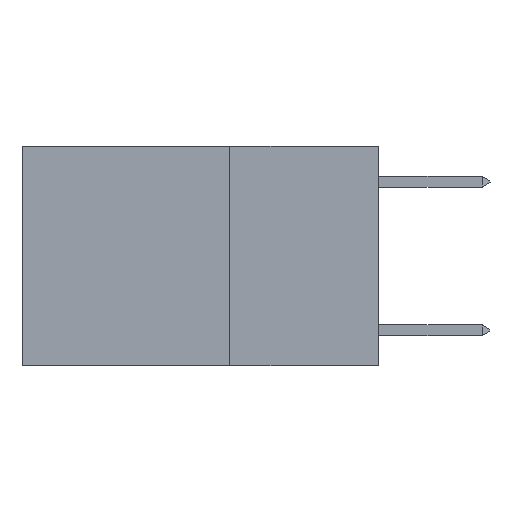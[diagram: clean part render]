
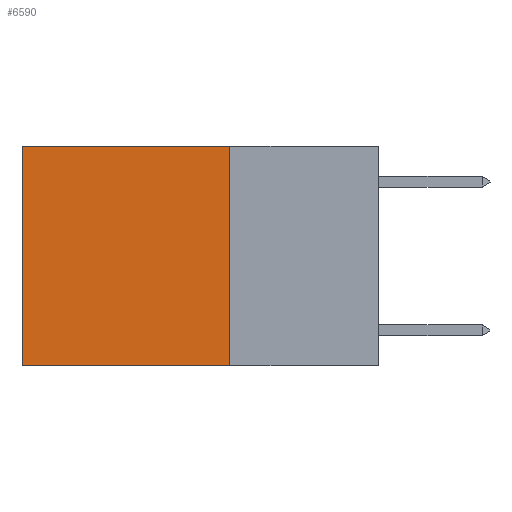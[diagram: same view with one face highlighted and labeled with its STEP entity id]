
A CAD part, left-side view. The second image highlights one B-rep face of the part: STEP entity #6590.
In plain terms, the highlighted planar face has unit normal (-1, 0, 0).
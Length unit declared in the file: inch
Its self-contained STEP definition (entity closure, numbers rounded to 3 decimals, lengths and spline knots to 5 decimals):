
#102 = LINE ( 'NONE', #12764, #19102 ) ;
#215 = EDGE_CURVE ( 'NONE', #3475, #6264, #17519, .T. ) ;
#253 = DIRECTION ( 'NONE',  ( 0., 0., -1. ) ) ;
#854 = LINE ( 'NONE', #14206, #12635 ) ;
#1300 = EDGE_LOOP ( 'NONE', ( #3783, #3819, #3892, #3922 ) ) ;
#2796 = CARTESIAN_POINT ( 'NONE',  ( 0.2625, 0.25, -0.37 ) ) ;
#3475 = VERTEX_POINT ( 'NONE', #7904 ) ;
#3783 = ORIENTED_EDGE ( 'NONE', *, *, #9590, .T. ) ;
#3819 = ORIENTED_EDGE ( 'NONE', *, *, #7355, .F. ) ;
#3892 = ORIENTED_EDGE ( 'NONE', *, *, #215, .F. ) ;
#3922 = ORIENTED_EDGE ( 'NONE', *, *, #8526, .T. ) ;
#4860 = FACE_OUTER_BOUND ( 'NONE', #1300, .T. ) ;
#5751 = DIRECTION ( 'NONE',  ( 0., 0., -1. ) ) ;
#6264 = VERTEX_POINT ( 'NONE', #2796 ) ;
#6590 = ADVANCED_FACE ( 'NONE', ( #4860 ), #16104, .F. ) ;
#7022 = CARTESIAN_POINT ( 'NONE',  ( 0.2625, 0.25, 0. ) ) ;
#7355 = EDGE_CURVE ( 'NONE', #6264, #15429, #854, .T. ) ;
#7838 = CARTESIAN_POINT ( 'NONE',  ( 0.2625, 0.25, 0. ) ) ;
#7904 = CARTESIAN_POINT ( 'NONE',  ( 0.2625, 0.25, 0. ) ) ;
#8027 = DIRECTION ( 'NONE',  ( 0., 1., 0. ) ) ;
#8526 = EDGE_CURVE ( 'NONE', #3475, #14657, #102, .T. ) ;
#8603 = DIRECTION ( 'NONE',  ( 1., 0., 0. ) ) ;
#9590 = EDGE_CURVE ( 'NONE', #14657, #15429, #19271, .T. ) ;
#11129 = VECTOR ( 'NONE', #5751, 39.37008 ) ;
#12266 = CARTESIAN_POINT ( 'NONE',  ( 0.2625, 0.6, -0.37 ) ) ;
#12592 = CARTESIAN_POINT ( 'NONE',  ( 0.2625, 0.6, 0. ) ) ;
#12635 = VECTOR ( 'NONE', #8027, 39.37008 ) ;
#12764 = CARTESIAN_POINT ( 'NONE',  ( 0.2625, 0.25, 0. ) ) ;
#13262 = VECTOR ( 'NONE', #253, 39.37008 ) ;
#14206 = CARTESIAN_POINT ( 'NONE',  ( 0.2625, 0.25, -0.37 ) ) ;
#14657 = VERTEX_POINT ( 'NONE', #12592 ) ;
#14951 = CARTESIAN_POINT ( 'NONE',  ( 0.2625, 0.6, 0. ) ) ;
#15429 = VERTEX_POINT ( 'NONE', #12266 ) ;
#15673 = DIRECTION ( 'NONE',  ( 0., 1., 0. ) ) ;
#16104 = PLANE ( 'NONE',  #19301 ) ;
#17519 = LINE ( 'NONE', #7838, #13262 ) ;
#18961 = DIRECTION ( 'NONE',  ( 0., 0., -1. ) ) ;
#19102 = VECTOR ( 'NONE', #15673, 39.37008 ) ;
#19271 = LINE ( 'NONE', #14951, #11129 ) ;
#19301 = AXIS2_PLACEMENT_3D ( 'NONE', #7022, #8603, #18961 ) ;
